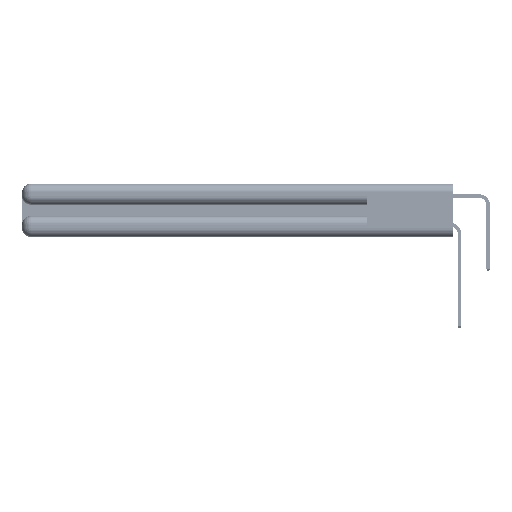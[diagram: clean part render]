
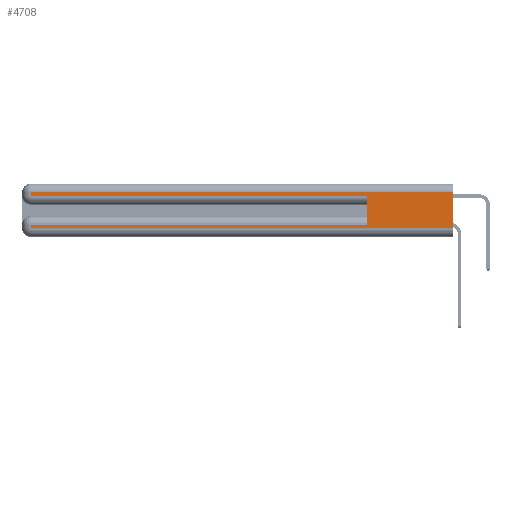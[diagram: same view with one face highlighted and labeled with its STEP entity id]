
A CAD part, left-side view. The second image highlights one B-rep face of the part: STEP entity #4708.
In plain terms, the highlighted planar face has unit normal (-1, 0, 0).
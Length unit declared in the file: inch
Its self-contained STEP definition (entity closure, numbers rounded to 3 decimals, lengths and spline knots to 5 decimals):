
#530 = CARTESIAN_POINT ( 'NONE',  ( 0., 2.94, 0.085 ) ) ;
#2750 = VECTOR ( 'NONE', #10835, 39.37008 ) ;
#3300 = VERTEX_POINT ( 'NONE', #530 ) ;
#4110 = VERTEX_POINT ( 'NONE', #29710 ) ;
#4708 = ADVANCED_FACE ( 'NONE', ( #13800 ), #9118, .F. ) ;
#6326 = CARTESIAN_POINT ( 'NONE',  ( 0., 2.94, 0.285 ) ) ;
#7118 = LINE ( 'NONE', #33733, #35146 ) ;
#7695 = CARTESIAN_POINT ( 'NONE',  ( 0., 2.94, 0.31 ) ) ;
#7710 = VERTEX_POINT ( 'NONE', #29197 ) ;
#9022 = LINE ( 'NONE', #48005, #22761 ) ;
#9118 = PLANE ( 'NONE',  #34921 ) ;
#10835 = DIRECTION ( 'NONE',  ( 0., 0., -1. ) ) ;
#11013 = CARTESIAN_POINT ( 'NONE',  ( 0., 2.94, 0.37 ) ) ;
#11465 = CARTESIAN_POINT ( 'NONE',  ( 0., 0., 0.285 ) ) ;
#11483 = EDGE_CURVE ( 'NONE', #7710, #3300, #24353, .T. ) ;
#11875 = ORIENTED_EDGE ( 'NONE', *, *, #43238, .T. ) ;
#11886 = EDGE_CURVE ( 'NONE', #4110, #24957, #50383, .T. ) ;
#11994 = CARTESIAN_POINT ( 'NONE',  ( 0., 0., 0.06 ) ) ;
#12157 = DIRECTION ( 'NONE',  ( 0., 1., 0. ) ) ;
#12638 = LINE ( 'NONE', #50898, #41842 ) ;
#13800 = FACE_OUTER_BOUND ( 'NONE', #19350, .T. ) ;
#14142 = VERTEX_POINT ( 'NONE', #7695 ) ;
#14238 = VERTEX_POINT ( 'NONE', #35711 ) ;
#15539 = ORIENTED_EDGE ( 'NONE', *, *, #17610, .T. ) ;
#16155 = ORIENTED_EDGE ( 'NONE', *, *, #35485, .F. ) ;
#17323 = DIRECTION ( 'NONE',  ( 1., 0., 0. ) ) ;
#17610 = EDGE_CURVE ( 'NONE', #48922, #14238, #31629, .T. ) ;
#17863 = DIRECTION ( 'NONE',  ( 0., 1., 0. ) ) ;
#18199 = CARTESIAN_POINT ( 'NONE',  ( 0., 0., 0.31 ) ) ;
#18339 = ORIENTED_EDGE ( 'NONE', *, *, #21273, .T. ) ;
#18490 = ORIENTED_EDGE ( 'NONE', *, *, #11886, .T. ) ;
#18930 = ORIENTED_EDGE ( 'NONE', *, *, #47082, .T. ) ;
#19350 = EDGE_LOOP ( 'NONE', ( #16155, #18339, #11875, #15539, #24394, #29915, #18930, #18490 ) ) ;
#21273 = EDGE_CURVE ( 'NONE', #29537, #14142, #48354, .T. ) ;
#22761 = VECTOR ( 'NONE', #40345, 39.37008 ) ;
#23095 = CARTESIAN_POINT ( 'NONE',  ( 0., 0., 0.06 ) ) ;
#23966 = LINE ( 'NONE', #11013, #2750 ) ;
#24353 = LINE ( 'NONE', #39825, #26824 ) ;
#24394 = ORIENTED_EDGE ( 'NONE', *, *, #30855, .F. ) ;
#24719 = VECTOR ( 'NONE', #17863, 39.37008 ) ;
#24957 = VERTEX_POINT ( 'NONE', #11994 ) ;
#25325 = CARTESIAN_POINT ( 'NONE',  ( 0., 0., 0.37 ) ) ;
#26824 = VECTOR ( 'NONE', #12157, 39.37008 ) ;
#27119 = DIRECTION ( 'NONE',  ( 0., -1., 0. ) ) ;
#28516 = VECTOR ( 'NONE', #27119, 39.37008 ) ;
#29197 = CARTESIAN_POINT ( 'NONE',  ( 0., 0.6, 0.085 ) ) ;
#29537 = VERTEX_POINT ( 'NONE', #34123 ) ;
#29710 = CARTESIAN_POINT ( 'NONE',  ( 0., 2.94, 0.06 ) ) ;
#29915 = ORIENTED_EDGE ( 'NONE', *, *, #11483, .T. ) ;
#30855 = EDGE_CURVE ( 'NONE', #7710, #14238, #12638, .T. ) ;
#31629 = LINE ( 'NONE', #11465, #28516 ) ;
#33733 = CARTESIAN_POINT ( 'NONE',  ( 0., 2.94, 0.37 ) ) ;
#33880 = DIRECTION ( 'NONE',  ( 0., -1., 0. ) ) ;
#34123 = CARTESIAN_POINT ( 'NONE',  ( 0., 0., 0.31 ) ) ;
#34921 = AXIS2_PLACEMENT_3D ( 'NONE', #25325, #17323, #41449 ) ;
#35146 = VECTOR ( 'NONE', #49893, 39.37008 ) ;
#35485 = EDGE_CURVE ( 'NONE', #29537, #24957, #9022, .T. ) ;
#35711 = CARTESIAN_POINT ( 'NONE',  ( 0., 0.6, 0.285 ) ) ;
#38418 = DIRECTION ( 'NONE',  ( 0., 0., 1. ) ) ;
#39825 = CARTESIAN_POINT ( 'NONE',  ( 0., 0., 0.085 ) ) ;
#40345 = DIRECTION ( 'NONE',  ( 0., 0., -1. ) ) ;
#41449 = DIRECTION ( 'NONE',  ( 0., 0., -1. ) ) ;
#41842 = VECTOR ( 'NONE', #38418, 39.37008 ) ;
#43238 = EDGE_CURVE ( 'NONE', #14142, #48922, #23966, .T. ) ;
#46660 = VECTOR ( 'NONE', #33880, 39.37008 ) ;
#47082 = EDGE_CURVE ( 'NONE', #3300, #4110, #7118, .T. ) ;
#48005 = CARTESIAN_POINT ( 'NONE',  ( 0., 0., 0.37 ) ) ;
#48354 = LINE ( 'NONE', #18199, #24719 ) ;
#48922 = VERTEX_POINT ( 'NONE', #6326 ) ;
#49893 = DIRECTION ( 'NONE',  ( 0., 0., -1. ) ) ;
#50383 = LINE ( 'NONE', #23095, #46660 ) ;
#50898 = CARTESIAN_POINT ( 'NONE',  ( 0., 0.6, 0.145 ) ) ;
